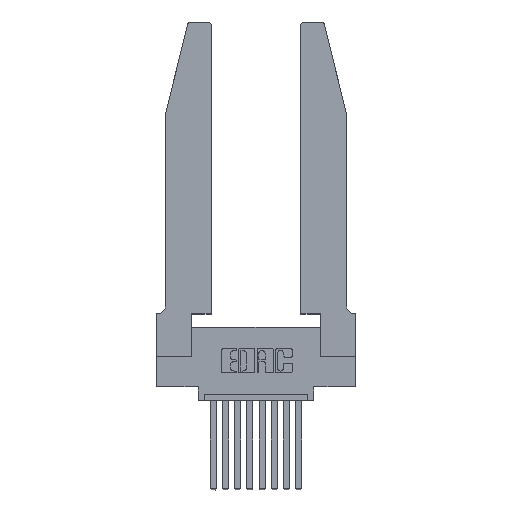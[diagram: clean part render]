
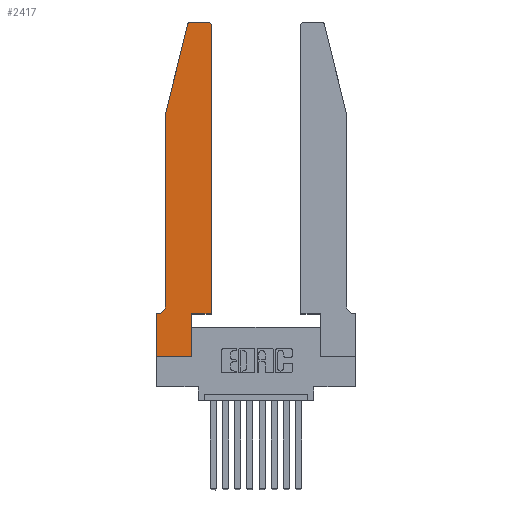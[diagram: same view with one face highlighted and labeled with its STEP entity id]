
A CAD part, top view. The second image highlights one B-rep face of the part: STEP entity #2417.
In plain terms, the highlighted planar face has unit normal (0, 0, 1).
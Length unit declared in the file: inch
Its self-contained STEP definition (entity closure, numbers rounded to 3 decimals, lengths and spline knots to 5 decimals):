
#8 = ORIENTED_EDGE ( 'NONE', *, *, #6964, .T. ) ;
#111 = CIRCLE ( 'NONE', #13122, 0.07 ) ;
#514 = DIRECTION ( 'NONE',  ( 1., 0., 0. ) ) ;
#522 = DIRECTION ( 'NONE',  ( -0.239, -0.971, 0. ) ) ;
#735 = CARTESIAN_POINT ( 'NONE',  ( 0., 0.35, 0.37 ) ) ;
#897 = CARTESIAN_POINT ( 'NONE',  ( 0.0055, 0.42, 0.37 ) ) ;
#926 = VECTOR ( 'NONE', #8566, 39.37008 ) ;
#1065 = CARTESIAN_POINT ( 'NONE',  ( 0.0755, 2., 0.37 ) ) ;
#1121 = EDGE_CURVE ( 'NONE', #1991, #10350, #4548, .T. ) ;
#1215 = EDGE_LOOP ( 'NONE', ( #8, #3493, #9674, #10887, #8149, #3151, #1915, #8301, #2582, #10065, #3778, #8595 ) ) ;
#1915 = ORIENTED_EDGE ( 'NONE', *, *, #12849, .T. ) ;
#1991 = VERTEX_POINT ( 'NONE', #7354 ) ;
#2301 = VECTOR ( 'NONE', #12854, 39.37008 ) ;
#2417 = ADVANCED_FACE ( 'NONE', ( #13326 ), #14359, .T. ) ;
#2582 = ORIENTED_EDGE ( 'NONE', *, *, #13624, .T. ) ;
#2592 = CARTESIAN_POINT ( 'NONE',  ( 0.2865, 0., 0.37 ) ) ;
#2612 = DIRECTION ( 'NONE',  ( 0., 0., 1. ) ) ;
#2852 = VERTEX_POINT ( 'NONE', #9927 ) ;
#2901 = AXIS2_PLACEMENT_3D ( 'NONE', #12680, #6888, #8062 ) ;
#3034 = DIRECTION ( 'NONE',  ( 0., 0., -1. ) ) ;
#3151 = ORIENTED_EDGE ( 'NONE', *, *, #13394, .T. ) ;
#3493 = ORIENTED_EDGE ( 'NONE', *, *, #10570, .T. ) ;
#3509 = CARTESIAN_POINT ( 'NONE',  ( 0.0755, 2., 0.37 ) ) ;
#3558 = VERTEX_POINT ( 'NONE', #2592 ) ;
#3623 = VECTOR ( 'NONE', #522, 39.37008 ) ;
#3739 = CIRCLE ( 'NONE', #2901, 0.03 ) ;
#3765 = DIRECTION ( 'NONE',  ( 0., 1., 0. ) ) ;
#3778 = ORIENTED_EDGE ( 'NONE', *, *, #12763, .T. ) ;
#4014 = VERTEX_POINT ( 'NONE', #9931 ) ;
#4044 = CARTESIAN_POINT ( 'NONE',  ( 0.25487, 2.72718, 0.37 ) ) ;
#4401 = AXIS2_PLACEMENT_3D ( 'NONE', #5418, #7790, #514 ) ;
#4446 = CARTESIAN_POINT ( 'NONE',  ( 0.2605, 2.75, 0.37 ) ) ;
#4489 = VERTEX_POINT ( 'NONE', #1065 ) ;
#4548 = LINE ( 'NONE', #4723, #2301 ) ;
#4723 = CARTESIAN_POINT ( 'NONE',  ( 0.4505, 0.35, 0.37 ) ) ;
#4730 = LINE ( 'NONE', #6705, #15216 ) ;
#5153 = DIRECTION ( 'NONE',  ( 1., 0., 0. ) ) ;
#5219 = CIRCLE ( 'NONE', #4401, 0.03 ) ;
#5418 = CARTESIAN_POINT ( 'NONE',  ( 0.284, 2.72, 0.37 ) ) ;
#5426 = EDGE_CURVE ( 'NONE', #4489, #5530, #11218, .T. ) ;
#5503 = EDGE_CURVE ( 'NONE', #5530, #4014, #111, .T. ) ;
#5530 = VERTEX_POINT ( 'NONE', #12337 ) ;
#5580 = DIRECTION ( 'NONE',  ( 0., -1., 0. ) ) ;
#5616 = DIRECTION ( 'NONE',  ( 0., -1., 0. ) ) ;
#5701 = DIRECTION ( 'NONE',  ( -1., 0., 0. ) ) ;
#5945 = VERTEX_POINT ( 'NONE', #14802 ) ;
#5956 = LINE ( 'NONE', #14555, #926 ) ;
#6165 = VERTEX_POINT ( 'NONE', #6246 ) ;
#6246 = CARTESIAN_POINT ( 'NONE',  ( 0.4505, 2.72, 0.37 ) ) ;
#6705 = CARTESIAN_POINT ( 'NONE',  ( 0.0755, 0.35, 0.37 ) ) ;
#6795 = VERTEX_POINT ( 'NONE', #7608 ) ;
#6834 = DIRECTION ( 'NONE',  ( 0., 1., 0. ) ) ;
#6888 = DIRECTION ( 'NONE',  ( 0., 0., 1. ) ) ;
#6957 = CARTESIAN_POINT ( 'NONE',  ( 0.0755, 2., 0.37 ) ) ;
#6964 = EDGE_CURVE ( 'NONE', #2852, #5945, #14305, .T. ) ;
#7163 = EDGE_CURVE ( 'NONE', #7982, #4489, #9881, .T. ) ;
#7283 = CARTESIAN_POINT ( 'NONE',  ( 0., 0.35, 0.37 ) ) ;
#7354 = CARTESIAN_POINT ( 'NONE',  ( 0.2865, 0.35, 0.37 ) ) ;
#7608 = CARTESIAN_POINT ( 'NONE',  ( 0., 0., 0.37 ) ) ;
#7790 = DIRECTION ( 'NONE',  ( 0., 0., 1. ) ) ;
#7844 = CARTESIAN_POINT ( 'NONE',  ( 0., 0., 0.37 ) ) ;
#7875 = LINE ( 'NONE', #12671, #12883 ) ;
#7982 = VERTEX_POINT ( 'NONE', #4044 ) ;
#8062 = DIRECTION ( 'NONE',  ( 1., 0., 0. ) ) ;
#8149 = ORIENTED_EDGE ( 'NONE', *, *, #5503, .T. ) ;
#8301 = ORIENTED_EDGE ( 'NONE', *, *, #10529, .T. ) ;
#8566 = DIRECTION ( 'NONE',  ( 1., 0., 0. ) ) ;
#8595 = ORIENTED_EDGE ( 'NONE', *, *, #9509, .T. ) ;
#8990 = VECTOR ( 'NONE', #5580, 39.37008 ) ;
#9509 = EDGE_CURVE ( 'NONE', #6165, #2852, #3739, .T. ) ;
#9521 = VECTOR ( 'NONE', #12697, 39.37008 ) ;
#9674 = ORIENTED_EDGE ( 'NONE', *, *, #7163, .T. ) ;
#9881 = LINE ( 'NONE', #3509, #3623 ) ;
#9927 = CARTESIAN_POINT ( 'NONE',  ( 0.4205, 2.75, 0.37 ) ) ;
#9931 = CARTESIAN_POINT ( 'NONE',  ( 0.0055, 0.35, 0.37 ) ) ;
#10065 = ORIENTED_EDGE ( 'NONE', *, *, #1121, .T. ) ;
#10304 = DIRECTION ( 'NONE',  ( -1., 0., 0. ) ) ;
#10350 = VERTEX_POINT ( 'NONE', #12030 ) ;
#10529 = EDGE_CURVE ( 'NONE', #6795, #3558, #5956, .T. ) ;
#10570 = EDGE_CURVE ( 'NONE', #5945, #7982, #5219, .T. ) ;
#10593 = VERTEX_POINT ( 'NONE', #735 ) ;
#10652 = VECTOR ( 'NONE', #5616, 39.37008 ) ;
#10887 = ORIENTED_EDGE ( 'NONE', *, *, #5426, .T. ) ;
#11218 = LINE ( 'NONE', #6957, #10652 ) ;
#12030 = CARTESIAN_POINT ( 'NONE',  ( 0.4505, 0.35, 0.37 ) ) ;
#12255 = LINE ( 'NONE', #14213, #13005 ) ;
#12337 = CARTESIAN_POINT ( 'NONE',  ( 0.0755, 0.42, 0.37 ) ) ;
#12507 = LINE ( 'NONE', #7844, #8990 ) ;
#12671 = CARTESIAN_POINT ( 'NONE',  ( 0.4505, 0.35, 0.37 ) ) ;
#12680 = CARTESIAN_POINT ( 'NONE',  ( 0.4205, 2.72, 0.37 ) ) ;
#12697 = DIRECTION ( 'NONE',  ( -1., 0., 0. ) ) ;
#12763 = EDGE_CURVE ( 'NONE', #10350, #6165, #7875, .T. ) ;
#12849 = EDGE_CURVE ( 'NONE', #10593, #6795, #12507, .T. ) ;
#12854 = DIRECTION ( 'NONE',  ( 1., 0., 0. ) ) ;
#12883 = VECTOR ( 'NONE', #6834, 39.37008 ) ;
#13005 = VECTOR ( 'NONE', #3765, 39.37008 ) ;
#13122 = AXIS2_PLACEMENT_3D ( 'NONE', #897, #3034, #5701 ) ;
#13326 = FACE_OUTER_BOUND ( 'NONE', #1215, .T. ) ;
#13394 = EDGE_CURVE ( 'NONE', #4014, #10593, #4730, .T. ) ;
#13624 = EDGE_CURVE ( 'NONE', #3558, #1991, #12255, .T. ) ;
#14213 = CARTESIAN_POINT ( 'NONE',  ( 0.2865, 0.35, 0.37 ) ) ;
#14305 = LINE ( 'NONE', #4446, #9521 ) ;
#14359 = PLANE ( 'NONE',  #15262 ) ;
#14555 = CARTESIAN_POINT ( 'NONE',  ( 0., 0., 0.37 ) ) ;
#14802 = CARTESIAN_POINT ( 'NONE',  ( 0.284, 2.75, 0.37 ) ) ;
#15216 = VECTOR ( 'NONE', #10304, 39.37008 ) ;
#15262 = AXIS2_PLACEMENT_3D ( 'NONE', #7283, #2612, #5153 ) ;
